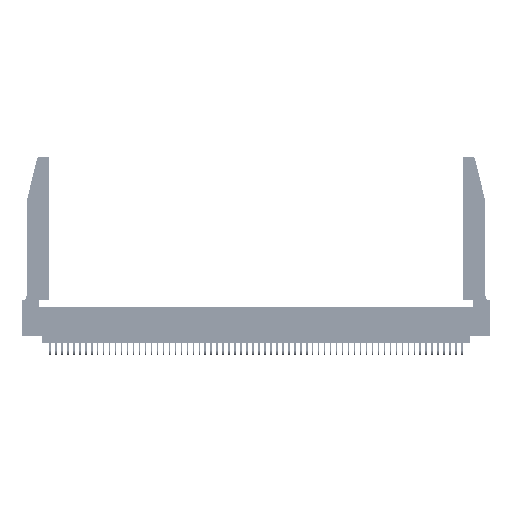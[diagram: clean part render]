
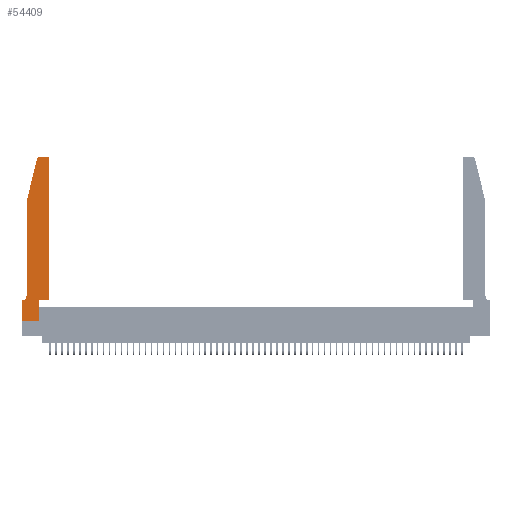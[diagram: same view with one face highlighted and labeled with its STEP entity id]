
A CAD part, top view. The second image highlights one B-rep face of the part: STEP entity #54409.
In plain terms, the highlighted planar face has unit normal (0, 0, 1).
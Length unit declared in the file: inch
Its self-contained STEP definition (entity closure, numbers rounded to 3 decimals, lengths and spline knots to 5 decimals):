
#424 = LINE ( 'NONE', #43921, #47867 ) ;
#502 = VERTEX_POINT ( 'NONE', #51864 ) ;
#539 = LINE ( 'NONE', #52531, #17230 ) ;
#896 = ORIENTED_EDGE ( 'NONE', *, *, #19803, .T. ) ;
#1552 = CARTESIAN_POINT ( 'NONE',  ( 0.0755, 2., 0.37 ) ) ;
#2107 = DIRECTION ( 'NONE',  ( 0., -1., 0. ) ) ;
#2558 = EDGE_CURVE ( 'NONE', #50878, #46140, #4335, .T. ) ;
#3137 = VERTEX_POINT ( 'NONE', #42444 ) ;
#3318 = EDGE_CURVE ( 'NONE', #14660, #43214, #21853, .T. ) ;
#3625 = VERTEX_POINT ( 'NONE', #18973 ) ;
#3945 = EDGE_CURVE ( 'NONE', #3625, #3137, #26659, .T. ) ;
#4127 = DIRECTION ( 'NONE',  ( 0., 1., 0. ) ) ;
#4335 = LINE ( 'NONE', #29024, #44813 ) ;
#4376 = CARTESIAN_POINT ( 'NONE',  ( 0.0055, 0.42, 0.37 ) ) ;
#5093 = DIRECTION ( 'NONE',  ( 1., 0., 0. ) ) ;
#5383 = EDGE_CURVE ( 'NONE', #46140, #14660, #47439, .T. ) ;
#5545 = ORIENTED_EDGE ( 'NONE', *, *, #46523, .T. ) ;
#6445 = EDGE_CURVE ( 'NONE', #3137, #29772, #539, .T. ) ;
#6645 = DIRECTION ( 'NONE',  ( 0., 0., 1. ) ) ;
#8517 = EDGE_LOOP ( 'NONE', ( #17033, #10865, #20299, #42210, #55682, #51828, #36389, #26377, #19887, #896, #46832, #5545 ) ) ;
#8849 = DIRECTION ( 'NONE',  ( 0., 0., -1. ) ) ;
#8878 = EDGE_CURVE ( 'NONE', #29772, #35942, #424, .T. ) ;
#9780 = CARTESIAN_POINT ( 'NONE',  ( 0.4205, 2.72, 0.37 ) ) ;
#10865 = ORIENTED_EDGE ( 'NONE', *, *, #31720, .T. ) ;
#11277 = DIRECTION ( 'NONE',  ( -0.239, -0.971, 0. ) ) ;
#11343 = CARTESIAN_POINT ( 'NONE',  ( 0.4505, 2.72, 0.37 ) ) ;
#11508 = CIRCLE ( 'NONE', #23646, 0.03 ) ;
#12493 = CARTESIAN_POINT ( 'NONE',  ( 0., 0., 0.37 ) ) ;
#12751 = DIRECTION ( 'NONE',  ( -1., 0., 0. ) ) ;
#13012 = CARTESIAN_POINT ( 'NONE',  ( 0.4505, 0.35, 0.37 ) ) ;
#13453 = LINE ( 'NONE', #52090, #55330 ) ;
#14660 = VERTEX_POINT ( 'NONE', #55932 ) ;
#14750 = VECTOR ( 'NONE', #22777, 39.37008 ) ;
#15195 = CARTESIAN_POINT ( 'NONE',  ( 0.2865, 0., 0.37 ) ) ;
#16148 = CARTESIAN_POINT ( 'NONE',  ( 0.2605, 2.75, 0.37 ) ) ;
#17033 = ORIENTED_EDGE ( 'NONE', *, *, #34225, .T. ) ;
#17230 = VECTOR ( 'NONE', #17784, 39.37008 ) ;
#17784 = DIRECTION ( 'NONE',  ( 1., 0., 0. ) ) ;
#18973 = CARTESIAN_POINT ( 'NONE',  ( 0., 0.35, 0.37 ) ) ;
#19600 = VERTEX_POINT ( 'NONE', #11343 ) ;
#19803 = EDGE_CURVE ( 'NONE', #35942, #33758, #13453, .T. ) ;
#19838 = CARTESIAN_POINT ( 'NONE',  ( 0.25487, 2.72718, 0.37 ) ) ;
#19887 = ORIENTED_EDGE ( 'NONE', *, *, #8878, .T. ) ;
#20299 = ORIENTED_EDGE ( 'NONE', *, *, #2558, .T. ) ;
#20469 = EDGE_CURVE ( 'NONE', #33758, #19600, #38522, .T. ) ;
#20501 = LINE ( 'NONE', #22972, #46358 ) ;
#20667 = CARTESIAN_POINT ( 'NONE',  ( 0.284, 2.72, 0.37 ) ) ;
#21285 = DIRECTION ( 'NONE',  ( 0., -1., 0. ) ) ;
#21853 = CIRCLE ( 'NONE', #39037, 0.07 ) ;
#22777 = DIRECTION ( 'NONE',  ( 0., 1., 0. ) ) ;
#22795 = VERTEX_POINT ( 'NONE', #49552 ) ;
#22972 = CARTESIAN_POINT ( 'NONE',  ( 0.0755, 0.35, 0.37 ) ) ;
#23646 = AXIS2_PLACEMENT_3D ( 'NONE', #20667, #6645, #56318 ) ;
#24754 = DIRECTION ( 'NONE',  ( -1., 0., 0. ) ) ;
#26216 = CARTESIAN_POINT ( 'NONE',  ( 0., 0.35, 0.37 ) ) ;
#26377 = ORIENTED_EDGE ( 'NONE', *, *, #6445, .T. ) ;
#26659 = LINE ( 'NONE', #12493, #44067 ) ;
#29024 = CARTESIAN_POINT ( 'NONE',  ( 0.0755, 2., 0.37 ) ) ;
#29772 = VERTEX_POINT ( 'NONE', #15195 ) ;
#31612 = DIRECTION ( 'NONE',  ( 1., 0., 0. ) ) ;
#31720 = EDGE_CURVE ( 'NONE', #502, #50878, #11508, .T. ) ;
#33758 = VERTEX_POINT ( 'NONE', #39445 ) ;
#34225 = EDGE_CURVE ( 'NONE', #22795, #502, #38523, .T. ) ;
#35942 = VERTEX_POINT ( 'NONE', #44496 ) ;
#36389 = ORIENTED_EDGE ( 'NONE', *, *, #3945, .T. ) ;
#36790 = EDGE_CURVE ( 'NONE', #43214, #3625, #20501, .T. ) ;
#38522 = LINE ( 'NONE', #13012, #14750 ) ;
#38523 = LINE ( 'NONE', #16148, #39175 ) ;
#39037 = AXIS2_PLACEMENT_3D ( 'NONE', #4376, #8849, #12751 ) ;
#39175 = VECTOR ( 'NONE', #24754, 39.37008 ) ;
#39315 = PLANE ( 'NONE',  #46796 ) ;
#39445 = CARTESIAN_POINT ( 'NONE',  ( 0.4505, 0.35, 0.37 ) ) ;
#41485 = DIRECTION ( 'NONE',  ( -1., 0., 0. ) ) ;
#42210 = ORIENTED_EDGE ( 'NONE', *, *, #5383, .T. ) ;
#42443 = AXIS2_PLACEMENT_3D ( 'NONE', #9780, #50155, #5093 ) ;
#42444 = CARTESIAN_POINT ( 'NONE',  ( 0., 0., 0.37 ) ) ;
#43211 = DIRECTION ( 'NONE',  ( 1., 0., 0. ) ) ;
#43214 = VERTEX_POINT ( 'NONE', #50813 ) ;
#43921 = CARTESIAN_POINT ( 'NONE',  ( 0.2865, 0.35, 0.37 ) ) ;
#44067 = VECTOR ( 'NONE', #21285, 39.37008 ) ;
#44496 = CARTESIAN_POINT ( 'NONE',  ( 0.2865, 0.35, 0.37 ) ) ;
#44813 = VECTOR ( 'NONE', #11277, 39.37008 ) ;
#46140 = VERTEX_POINT ( 'NONE', #46683 ) ;
#46358 = VECTOR ( 'NONE', #41485, 39.37008 ) ;
#46523 = EDGE_CURVE ( 'NONE', #19600, #22795, #47921, .T. ) ;
#46683 = CARTESIAN_POINT ( 'NONE',  ( 0.0755, 2., 0.37 ) ) ;
#46796 = AXIS2_PLACEMENT_3D ( 'NONE', #26216, #48270, #43211 ) ;
#46832 = ORIENTED_EDGE ( 'NONE', *, *, #20469, .T. ) ;
#47439 = LINE ( 'NONE', #1552, #55748 ) ;
#47867 = VECTOR ( 'NONE', #4127, 39.37008 ) ;
#47921 = CIRCLE ( 'NONE', #42443, 0.03 ) ;
#48270 = DIRECTION ( 'NONE',  ( 0., 0., 1. ) ) ;
#49552 = CARTESIAN_POINT ( 'NONE',  ( 0.4205, 2.75, 0.37 ) ) ;
#50155 = DIRECTION ( 'NONE',  ( 0., 0., 1. ) ) ;
#50813 = CARTESIAN_POINT ( 'NONE',  ( 0.0055, 0.35, 0.37 ) ) ;
#50878 = VERTEX_POINT ( 'NONE', #19838 ) ;
#51828 = ORIENTED_EDGE ( 'NONE', *, *, #36790, .T. ) ;
#51864 = CARTESIAN_POINT ( 'NONE',  ( 0.284, 2.75, 0.37 ) ) ;
#52090 = CARTESIAN_POINT ( 'NONE',  ( 0.4505, 0.35, 0.37 ) ) ;
#52531 = CARTESIAN_POINT ( 'NONE',  ( 0., 0., 0.37 ) ) ;
#54409 = ADVANCED_FACE ( 'NONE', ( #57483 ), #39315, .T. ) ;
#55330 = VECTOR ( 'NONE', #31612, 39.37008 ) ;
#55682 = ORIENTED_EDGE ( 'NONE', *, *, #3318, .T. ) ;
#55748 = VECTOR ( 'NONE', #2107, 39.37008 ) ;
#55932 = CARTESIAN_POINT ( 'NONE',  ( 0.0755, 0.42, 0.37 ) ) ;
#56318 = DIRECTION ( 'NONE',  ( 1., 0., 0. ) ) ;
#57483 = FACE_OUTER_BOUND ( 'NONE', #8517, .T. ) ;
